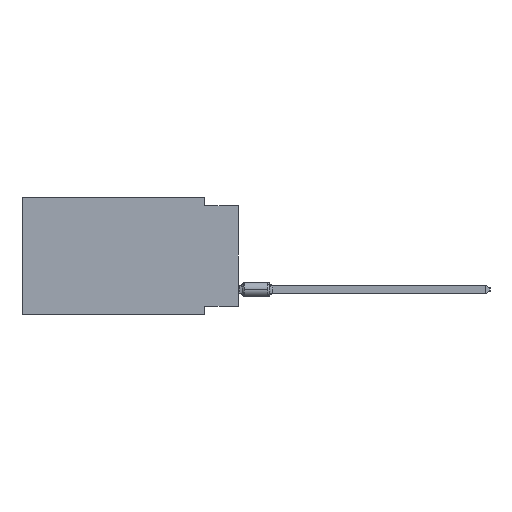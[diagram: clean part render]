
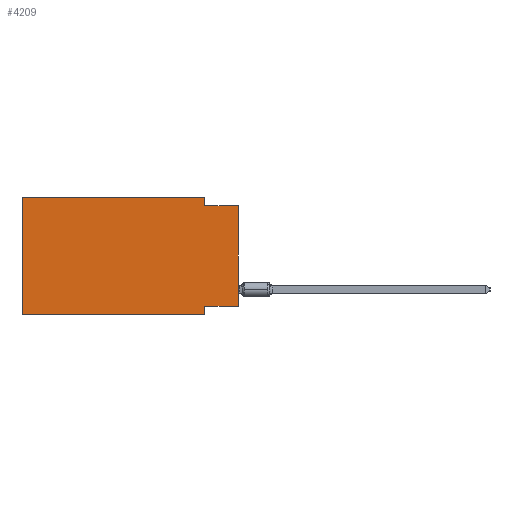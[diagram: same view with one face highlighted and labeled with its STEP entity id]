
A CAD part, left-side view. The second image highlights one B-rep face of the part: STEP entity #4209.
In plain terms, the highlighted planar face has unit normal (-1, 0, 0).
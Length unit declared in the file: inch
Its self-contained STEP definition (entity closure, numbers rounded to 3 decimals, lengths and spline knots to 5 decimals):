
#963 = DIRECTION ( 'NONE',  ( 0., -1., 0. ) ) ;
#1446 = EDGE_LOOP ( 'NONE', ( #10064, #19777, #7768, #10545, #17435, #3567, #7305, #7831 ) ) ;
#2030 = LINE ( 'NONE', #16067, #5094 ) ;
#2440 = CARTESIAN_POINT ( 'NONE',  ( 0., 0.645, 0. ) ) ;
#2821 = LINE ( 'NONE', #13407, #19763 ) ;
#3237 = PLANE ( 'NONE',  #17715 ) ;
#3567 = ORIENTED_EDGE ( 'NONE', *, *, #12326, .T. ) ;
#3632 = EDGE_CURVE ( 'NONE', #14168, #22032, #22046, .T. ) ;
#4202 = VERTEX_POINT ( 'NONE', #10020 ) ;
#4209 = ADVANCED_FACE ( 'NONE', ( #9789 ), #3237, .F. ) ;
#4247 = VECTOR ( 'NONE', #11205, 39.37008 ) ;
#4942 = EDGE_CURVE ( 'NONE', #19150, #6899, #16619, .T. ) ;
#5094 = VECTOR ( 'NONE', #17688, 39.37008 ) ;
#5716 = CARTESIAN_POINT ( 'NONE',  ( 0., 0.1, -0.325 ) ) ;
#6834 = CARTESIAN_POINT ( 'NONE',  ( 0., 0., -0.325 ) ) ;
#6899 = VERTEX_POINT ( 'NONE', #18669 ) ;
#7047 = CARTESIAN_POINT ( 'NONE',  ( 0., 0.1, -0.025 ) ) ;
#7305 = ORIENTED_EDGE ( 'NONE', *, *, #12276, .F. ) ;
#7434 = VERTEX_POINT ( 'NONE', #5716 ) ;
#7768 = ORIENTED_EDGE ( 'NONE', *, *, #9035, .F. ) ;
#7781 = CARTESIAN_POINT ( 'NONE',  ( 0., 0.1, -0.35 ) ) ;
#7831 = ORIENTED_EDGE ( 'NONE', *, *, #11202, .F. ) ;
#8140 = VECTOR ( 'NONE', #13630, 39.37008 ) ;
#8187 = CARTESIAN_POINT ( 'NONE',  ( 0., 0., 0. ) ) ;
#8345 = VECTOR ( 'NONE', #16825, 39.37008 ) ;
#8941 = VERTEX_POINT ( 'NONE', #13763 ) ;
#9035 = EDGE_CURVE ( 'NONE', #6899, #14168, #2030, .T. ) ;
#9455 = DIRECTION ( 'NONE',  ( 0., 0., 1. ) ) ;
#9685 = EDGE_CURVE ( 'NONE', #4202, #22032, #20737, .T. ) ;
#9687 = CARTESIAN_POINT ( 'NONE',  ( 0., 0., -0.025 ) ) ;
#9706 = CARTESIAN_POINT ( 'NONE',  ( 0., 0.645, 0. ) ) ;
#9789 = FACE_OUTER_BOUND ( 'NONE', #1446, .T. ) ;
#9831 = DIRECTION ( 'NONE',  ( 0., -1., 0. ) ) ;
#9854 = VECTOR ( 'NONE', #9455, 39.37008 ) ;
#10020 = CARTESIAN_POINT ( 'NONE',  ( 0., 0., -0.325 ) ) ;
#10064 = ORIENTED_EDGE ( 'NONE', *, *, #9685, .T. ) ;
#10418 = VECTOR ( 'NONE', #963, 39.37008 ) ;
#10545 = ORIENTED_EDGE ( 'NONE', *, *, #4942, .F. ) ;
#11202 = EDGE_CURVE ( 'NONE', #4202, #7434, #17203, .T. ) ;
#11205 = DIRECTION ( 'NONE',  ( 0., -1., 0. ) ) ;
#11636 = DIRECTION ( 'NONE',  ( 1., 0., 0. ) ) ;
#11870 = DIRECTION ( 'NONE',  ( 0., 0., -1. ) ) ;
#12276 = EDGE_CURVE ( 'NONE', #7434, #8941, #14801, .T. ) ;
#12326 = EDGE_CURVE ( 'NONE', #19391, #8941, #2821, .T. ) ;
#13256 = CARTESIAN_POINT ( 'NONE',  ( 0., 0.645, 0. ) ) ;
#13278 = CARTESIAN_POINT ( 'NONE',  ( 0., 0., -0.025 ) ) ;
#13407 = CARTESIAN_POINT ( 'NONE',  ( 0., 0.645, -0.35 ) ) ;
#13511 = VECTOR ( 'NONE', #16635, 39.37008 ) ;
#13630 = DIRECTION ( 'NONE',  ( 0., 1., 0. ) ) ;
#13763 = CARTESIAN_POINT ( 'NONE',  ( 0., 0.1, -0.35 ) ) ;
#14168 = VERTEX_POINT ( 'NONE', #7047 ) ;
#14281 = CARTESIAN_POINT ( 'NONE',  ( 0., 0.645, -0.35 ) ) ;
#14421 = CARTESIAN_POINT ( 'NONE',  ( 0., 0.645, 0. ) ) ;
#14801 = LINE ( 'NONE', #7781, #13511 ) ;
#16067 = CARTESIAN_POINT ( 'NONE',  ( 0., 0.1, 0. ) ) ;
#16619 = LINE ( 'NONE', #9706, #4247 ) ;
#16635 = DIRECTION ( 'NONE',  ( 0., 0., -1. ) ) ;
#16825 = DIRECTION ( 'NONE',  ( 0., 0., 1. ) ) ;
#17203 = LINE ( 'NONE', #6834, #8140 ) ;
#17435 = ORIENTED_EDGE ( 'NONE', *, *, #19228, .F. ) ;
#17688 = DIRECTION ( 'NONE',  ( 0., 0., -1. ) ) ;
#17715 = AXIS2_PLACEMENT_3D ( 'NONE', #13256, #11636, #11870 ) ;
#18669 = CARTESIAN_POINT ( 'NONE',  ( 0., 0.1, 0. ) ) ;
#19150 = VERTEX_POINT ( 'NONE', #14421 ) ;
#19228 = EDGE_CURVE ( 'NONE', #19391, #19150, #20039, .T. ) ;
#19391 = VERTEX_POINT ( 'NONE', #14281 ) ;
#19763 = VECTOR ( 'NONE', #9831, 39.37008 ) ;
#19777 = ORIENTED_EDGE ( 'NONE', *, *, #3632, .F. ) ;
#20039 = LINE ( 'NONE', #2440, #9854 ) ;
#20737 = LINE ( 'NONE', #8187, #8345 ) ;
#22032 = VERTEX_POINT ( 'NONE', #9687 ) ;
#22046 = LINE ( 'NONE', #13278, #10418 ) ;
